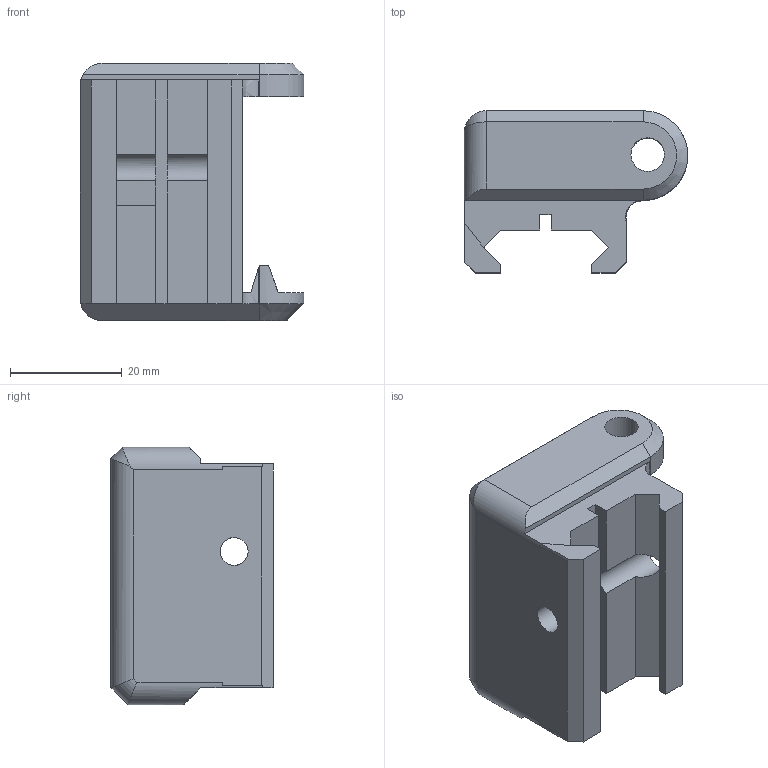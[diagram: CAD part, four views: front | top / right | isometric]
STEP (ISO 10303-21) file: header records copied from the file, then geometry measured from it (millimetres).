
FILE_DESCRIPTION(/* description */ (''),/* implementation_level */ '2;1');
FILE_NAME(/* name */ 'Brace Hinge.step',/* time_stamp */ '2021-01-18T14:15:57-07:00',/* author */ (''),/* organization */ (''),/* preprocessor_version */ 'ST-DEVELOPER v18.1',/* originating_system */ 'Autodesk Translation Framework v9.7.1.1290',/* authorisation */ '');
FILE_SCHEMA (('AUTOMOTIVE_DESIGN { 1 0 10303 214 3 1 1 }'));
Length unit declared in the file: inch
Products named in the file (1): Space Gun Beta Ready
Bounding box: 40 x 28.99 x 46 mm (x, y, z)
Volume: 16783 mm3; surface area: 8897 mm2
Topology: 1 solids, 1 shells, 97 faces, 285 edges, 187 vertices
Faces by surface type: plane 81, cylinder 12, bspline 2, cone 2
Full cylindrical faces by diameter (mm): 5 x2, 6 x2
Entity records: 3442 total; most frequent: CARTESIAN_POINT 751, ORIENTED_EDGE 570, DIRECTION 532, EDGE_CURVE 285, LINE 216, VECTOR 216, VERTEX_POINT 187, AXIS2_PLACEMENT_3D 158
